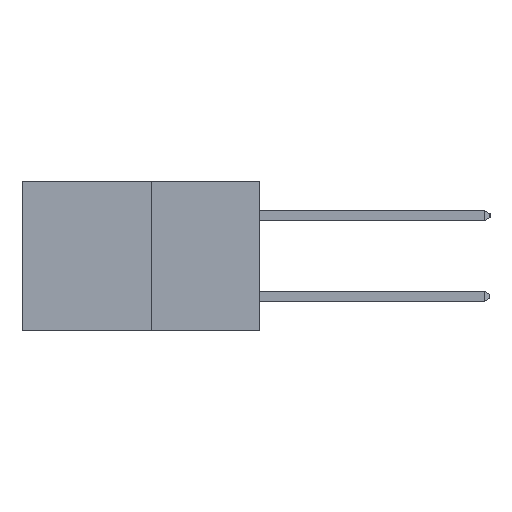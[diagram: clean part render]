
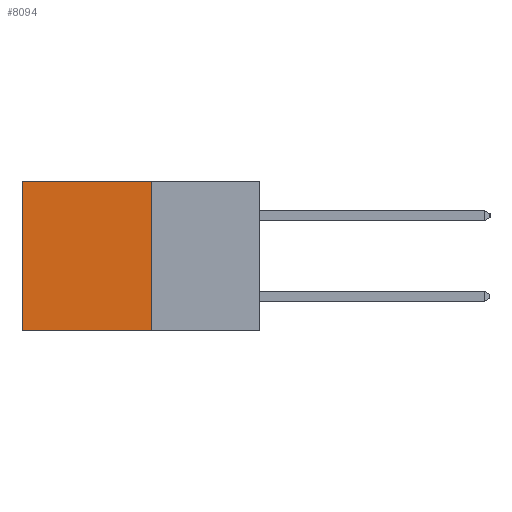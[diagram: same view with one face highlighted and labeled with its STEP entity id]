
A CAD part, left-side view. The second image highlights one B-rep face of the part: STEP entity #8094.
In plain terms, the highlighted planar face has unit normal (-1, 0, 0).
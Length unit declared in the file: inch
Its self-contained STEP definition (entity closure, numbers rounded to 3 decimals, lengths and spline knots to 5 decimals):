
#1384 = DIRECTION ( 'NONE',  ( 0., 1., 0. ) ) ;
#1469 = CARTESIAN_POINT ( 'NONE',  ( 0.277, 0.27, 0. ) ) ;
#1492 = CARTESIAN_POINT ( 'NONE',  ( 0.277, 0.27, 0. ) ) ;
#2514 = EDGE_LOOP ( 'NONE', ( #10301, #8921, #4089, #7631 ) ) ;
#2762 = CARTESIAN_POINT ( 'NONE',  ( 0.277, 0.59, -0.37 ) ) ;
#2818 = EDGE_CURVE ( 'NONE', #10318, #5537, #9105, .T. ) ;
#3828 = AXIS2_PLACEMENT_3D ( 'NONE', #11255, #5442, #12190 ) ;
#4089 = ORIENTED_EDGE ( 'NONE', *, *, #10936, .F. ) ;
#4106 = DIRECTION ( 'NONE',  ( 0., 0., -1. ) ) ;
#4340 = LINE ( 'NONE', #5837, #11526 ) ;
#4440 = PLANE ( 'NONE',  #3828 ) ;
#5442 = DIRECTION ( 'NONE',  ( 1., 0., 0. ) ) ;
#5537 = VERTEX_POINT ( 'NONE', #6197 ) ;
#5837 = CARTESIAN_POINT ( 'NONE',  ( 0.277, 0.59, -0.37 ) ) ;
#5956 = VERTEX_POINT ( 'NONE', #6950 ) ;
#6197 = CARTESIAN_POINT ( 'NONE',  ( 0.277, 0.59, 0. ) ) ;
#6307 = EDGE_CURVE ( 'NONE', #5956, #8318, #7262, .T. ) ;
#6422 = VECTOR ( 'NONE', #1384, 39.37008 ) ;
#6762 = FACE_OUTER_BOUND ( 'NONE', #2514, .T. ) ;
#6808 = EDGE_CURVE ( 'NONE', #5537, #8318, #4340, .T. ) ;
#6950 = CARTESIAN_POINT ( 'NONE',  ( 0.277, 0.27, -0.37 ) ) ;
#7262 = LINE ( 'NONE', #7918, #9314 ) ;
#7631 = ORIENTED_EDGE ( 'NONE', *, *, #2818, .T. ) ;
#7918 = CARTESIAN_POINT ( 'NONE',  ( 0.277, 0.27, -0.37 ) ) ;
#8094 = ADVANCED_FACE ( 'NONE', ( #6762 ), #4440, .F. ) ;
#8318 = VERTEX_POINT ( 'NONE', #2762 ) ;
#8921 = ORIENTED_EDGE ( 'NONE', *, *, #6307, .F. ) ;
#8940 = DIRECTION ( 'NONE',  ( 0., 1., 0. ) ) ;
#9105 = LINE ( 'NONE', #1492, #6422 ) ;
#9314 = VECTOR ( 'NONE', #8940, 39.37008 ) ;
#10301 = ORIENTED_EDGE ( 'NONE', *, *, #6808, .T. ) ;
#10318 = VERTEX_POINT ( 'NONE', #1469 ) ;
#10936 = EDGE_CURVE ( 'NONE', #10318, #5956, #11894, .T. ) ;
#10986 = CARTESIAN_POINT ( 'NONE',  ( 0.277, 0.27, -0.37 ) ) ;
#11255 = CARTESIAN_POINT ( 'NONE',  ( 0.277, 0.27, -0.37 ) ) ;
#11514 = DIRECTION ( 'NONE',  ( 0., 0., -1. ) ) ;
#11526 = VECTOR ( 'NONE', #11514, 39.37008 ) ;
#11894 = LINE ( 'NONE', #10986, #12159 ) ;
#12159 = VECTOR ( 'NONE', #4106, 39.37008 ) ;
#12190 = DIRECTION ( 'NONE',  ( 0., 0., -1. ) ) ;
